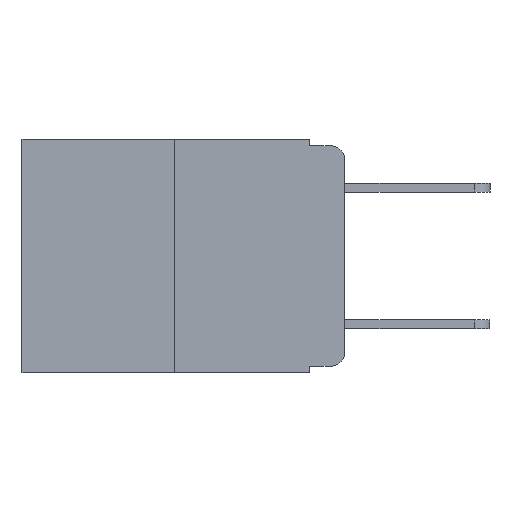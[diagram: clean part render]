
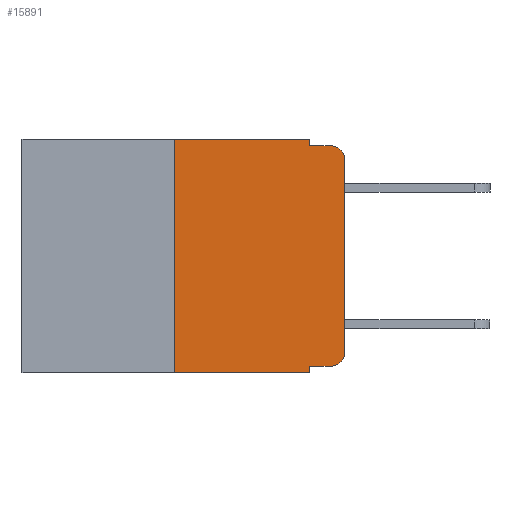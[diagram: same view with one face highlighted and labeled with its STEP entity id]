
A CAD part, left-side view. The second image highlights one B-rep face of the part: STEP entity #15891.
In plain terms, the highlighted planar face has unit normal (-1, 0, 0).
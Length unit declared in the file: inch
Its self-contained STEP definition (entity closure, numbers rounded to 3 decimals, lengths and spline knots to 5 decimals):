
#426 = VERTEX_POINT ( 'NONE', #4268 ) ;
#784 = PLANE ( 'NONE',  #17718 ) ;
#2071 = LINE ( 'NONE', #5253, #5728 ) ;
#2808 = VERTEX_POINT ( 'NONE', #9987 ) ;
#2848 = VECTOR ( 'NONE', #21375, 39.37008 ) ;
#3012 = CARTESIAN_POINT ( 'NONE',  ( 0., 0., -0.313 ) ) ;
#3198 = ORIENTED_EDGE ( 'NONE', *, *, #4943, .T. ) ;
#3279 = CARTESIAN_POINT ( 'NONE',  ( 0., 0.25, 0. ) ) ;
#3317 = ORIENTED_EDGE ( 'NONE', *, *, #12962, .T. ) ;
#3469 = EDGE_CURVE ( 'NONE', #9529, #426, #11047, .T. ) ;
#3856 = DIRECTION ( 'NONE',  ( -1., 0., 0. ) ) ;
#3942 = FACE_OUTER_BOUND ( 'NONE', #14015, .T. ) ;
#4024 = CARTESIAN_POINT ( 'NONE',  ( 0., 0.02, -0.03 ) ) ;
#4216 = VECTOR ( 'NONE', #5100, 39.37008 ) ;
#4268 = CARTESIAN_POINT ( 'NONE',  ( 0., 0., -0.03 ) ) ;
#4409 = DIRECTION ( 'NONE',  ( 1., 0., 0. ) ) ;
#4943 = EDGE_CURVE ( 'NONE', #426, #2808, #20173, .T. ) ;
#5067 = CARTESIAN_POINT ( 'NONE',  ( 0., 0.051, 0. ) ) ;
#5100 = DIRECTION ( 'NONE',  ( 0., 0., 1. ) ) ;
#5253 = CARTESIAN_POINT ( 'NONE',  ( 0., 0.051, 0. ) ) ;
#5379 = VECTOR ( 'NONE', #23545, 39.37008 ) ;
#5728 = VECTOR ( 'NONE', #21683, 39.37008 ) ;
#5752 = LINE ( 'NONE', #5831, #19725 ) ;
#5831 = CARTESIAN_POINT ( 'NONE',  ( 0., 0.051, 0. ) ) ;
#5840 = DIRECTION ( 'NONE',  ( 0., 0., -1. ) ) ;
#5996 = VERTEX_POINT ( 'NONE', #8659 ) ;
#6018 = VERTEX_POINT ( 'NONE', #12249 ) ;
#6278 = VECTOR ( 'NONE', #10029, 39.37008 ) ;
#6646 = ORIENTED_EDGE ( 'NONE', *, *, #22088, .F. ) ;
#6647 = VECTOR ( 'NONE', #22903, 39.37008 ) ;
#6747 = ORIENTED_EDGE ( 'NONE', *, *, #9791, .T. ) ;
#7241 = ORIENTED_EDGE ( 'NONE', *, *, #16133, .F. ) ;
#7637 = VERTEX_POINT ( 'NONE', #15870 ) ;
#7647 = LINE ( 'NONE', #15796, #2848 ) ;
#7779 = CIRCLE ( 'NONE', #19501, 0.02 ) ;
#8290 = ORIENTED_EDGE ( 'NONE', *, *, #3469, .T. ) ;
#8659 = CARTESIAN_POINT ( 'NONE',  ( 0., 0.051, -0.343 ) ) ;
#8749 = CARTESIAN_POINT ( 'NONE',  ( 0., 0.051, -0.01 ) ) ;
#9051 = LINE ( 'NONE', #9956, #10147 ) ;
#9493 = AXIS2_PLACEMENT_3D ( 'NONE', #4024, #16704, #5840 ) ;
#9529 = VERTEX_POINT ( 'NONE', #3012 ) ;
#9791 = EDGE_CURVE ( 'NONE', #20486, #9529, #7779, .T. ) ;
#9956 = CARTESIAN_POINT ( 'NONE',  ( 0., 0.051, -0.333 ) ) ;
#9987 = CARTESIAN_POINT ( 'NONE',  ( 0., 0.02, -0.01 ) ) ;
#10029 = DIRECTION ( 'NONE',  ( 0., 0., 1. ) ) ;
#10147 = VECTOR ( 'NONE', #11983, 39.37008 ) ;
#10231 = EDGE_CURVE ( 'NONE', #16894, #18641, #11414, .T. ) ;
#10620 = ORIENTED_EDGE ( 'NONE', *, *, #15601, .T. ) ;
#11047 = LINE ( 'NONE', #22679, #6278 ) ;
#11414 = LINE ( 'NONE', #11910, #6647 ) ;
#11910 = CARTESIAN_POINT ( 'NONE',  ( 0., 0.473, 0. ) ) ;
#11983 = DIRECTION ( 'NONE',  ( 0., -1., 0. ) ) ;
#12249 = CARTESIAN_POINT ( 'NONE',  ( 0., 0.051, -0.333 ) ) ;
#12962 = EDGE_CURVE ( 'NONE', #6018, #20486, #9051, .T. ) ;
#13481 = ORIENTED_EDGE ( 'NONE', *, *, #22522, .F. ) ;
#14015 = EDGE_LOOP ( 'NONE', ( #8290, #3198, #17145, #6646, #17748, #7241, #10620, #13481, #3317, #6747 ) ) ;
#14711 = CARTESIAN_POINT ( 'NONE',  ( 0., 0.02, -0.313 ) ) ;
#15256 = CARTESIAN_POINT ( 'NONE',  ( 0., 0.02, -0.333 ) ) ;
#15265 = CARTESIAN_POINT ( 'NONE',  ( 0., 0.473, 0. ) ) ;
#15464 = EDGE_CURVE ( 'NONE', #18868, #2808, #7647, .T. ) ;
#15601 = EDGE_CURVE ( 'NONE', #7637, #5996, #19923, .T. ) ;
#15796 = CARTESIAN_POINT ( 'NONE',  ( 0., 0.051, -0.01 ) ) ;
#15870 = CARTESIAN_POINT ( 'NONE',  ( 0., 0.25, -0.343 ) ) ;
#15891 = ADVANCED_FACE ( 'NONE', ( #3942 ), #784, .F. ) ;
#16133 = EDGE_CURVE ( 'NONE', #7637, #16894, #18737, .T. ) ;
#16557 = DIRECTION ( 'NONE',  ( 0., 0., -1. ) ) ;
#16687 = DIRECTION ( 'NONE',  ( 0., 0., -1. ) ) ;
#16704 = DIRECTION ( 'NONE',  ( -1., 0., 0. ) ) ;
#16894 = VERTEX_POINT ( 'NONE', #23531 ) ;
#17118 = DIRECTION ( 'NONE',  ( 0., 0., -1. ) ) ;
#17145 = ORIENTED_EDGE ( 'NONE', *, *, #15464, .F. ) ;
#17718 = AXIS2_PLACEMENT_3D ( 'NONE', #15265, #4409, #17118 ) ;
#17748 = ORIENTED_EDGE ( 'NONE', *, *, #10231, .F. ) ;
#18035 = CARTESIAN_POINT ( 'NONE',  ( 0., 0.473, -0.343 ) ) ;
#18641 = VERTEX_POINT ( 'NONE', #5067 ) ;
#18737 = LINE ( 'NONE', #3279, #4216 ) ;
#18868 = VERTEX_POINT ( 'NONE', #8749 ) ;
#19501 = AXIS2_PLACEMENT_3D ( 'NONE', #14711, #3856, #16557 ) ;
#19725 = VECTOR ( 'NONE', #16687, 39.37008 ) ;
#19923 = LINE ( 'NONE', #18035, #5379 ) ;
#20173 = CIRCLE ( 'NONE', #9493, 0.02 ) ;
#20486 = VERTEX_POINT ( 'NONE', #15256 ) ;
#21375 = DIRECTION ( 'NONE',  ( 0., -1., 0. ) ) ;
#21683 = DIRECTION ( 'NONE',  ( 0., 0., -1. ) ) ;
#22088 = EDGE_CURVE ( 'NONE', #18641, #18868, #5752, .T. ) ;
#22522 = EDGE_CURVE ( 'NONE', #6018, #5996, #2071, .T. ) ;
#22679 = CARTESIAN_POINT ( 'NONE',  ( 0., 0., 0. ) ) ;
#22903 = DIRECTION ( 'NONE',  ( 0., -1., 0. ) ) ;
#23531 = CARTESIAN_POINT ( 'NONE',  ( 0., 0.25, 0. ) ) ;
#23545 = DIRECTION ( 'NONE',  ( 0., -1., 0. ) ) ;
